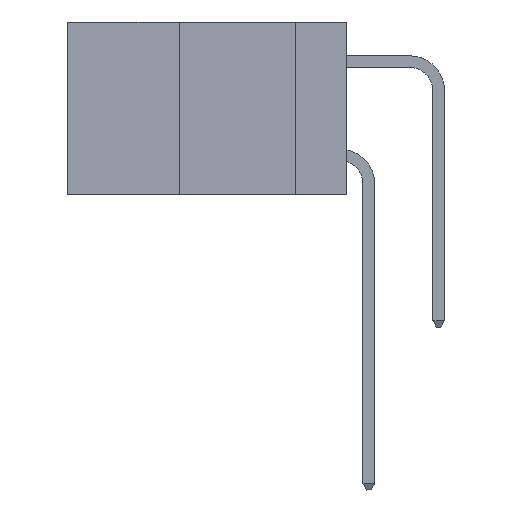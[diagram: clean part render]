
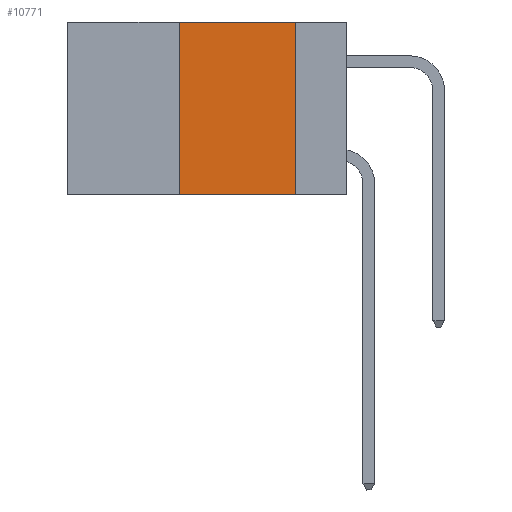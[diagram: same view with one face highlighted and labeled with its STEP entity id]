
A CAD part, left-side view. The second image highlights one B-rep face of the part: STEP entity #10771.
In plain terms, the highlighted planar face has unit normal (-1, 0, 0).
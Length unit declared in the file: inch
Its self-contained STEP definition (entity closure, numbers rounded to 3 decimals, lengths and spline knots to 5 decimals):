
#454 = VERTEX_POINT ( 'NONE', #17388 ) ;
#482 = PLANE ( 'NONE',  #4705 ) ;
#627 = EDGE_CURVE ( 'NONE', #16099, #19347, #20207, .T. ) ;
#819 = CARTESIAN_POINT ( 'NONE',  ( 0., 0.11, 0. ) ) ;
#1602 = CARTESIAN_POINT ( 'NONE',  ( 0., 0.11, -0.37 ) ) ;
#1875 = DIRECTION ( 'NONE',  ( 0., -1., 0. ) ) ;
#2126 = VECTOR ( 'NONE', #21507, 39.37008 ) ;
#2266 = DIRECTION ( 'NONE',  ( 1., 0., 0. ) ) ;
#2943 = EDGE_CURVE ( 'NONE', #454, #19347, #16893, .T. ) ;
#3566 = CARTESIAN_POINT ( 'NONE',  ( 0., 0.11, 0. ) ) ;
#4705 = AXIS2_PLACEMENT_3D ( 'NONE', #15575, #2266, #18907 ) ;
#5566 = ORIENTED_EDGE ( 'NONE', *, *, #17173, .F. ) ;
#5903 = ORIENTED_EDGE ( 'NONE', *, *, #627, .F. ) ;
#6256 = CARTESIAN_POINT ( 'NONE',  ( 0., 0.6, -0.37 ) ) ;
#6692 = LINE ( 'NONE', #11404, #2126 ) ;
#7516 = VECTOR ( 'NONE', #7964, 39.37008 ) ;
#7964 = DIRECTION ( 'NONE',  ( 0., -1., 0. ) ) ;
#8406 = FACE_OUTER_BOUND ( 'NONE', #18577, .T. ) ;
#9780 = ORIENTED_EDGE ( 'NONE', *, *, #2943, .T. ) ;
#10770 = VECTOR ( 'NONE', #16052, 39.37008 ) ;
#10771 = ADVANCED_FACE ( 'NONE', ( #8406 ), #482, .F. ) ;
#11404 = CARTESIAN_POINT ( 'NONE',  ( 0., 0.36, 0. ) ) ;
#13070 = LINE ( 'NONE', #13634, #14631 ) ;
#13322 = EDGE_CURVE ( 'NONE', #454, #16764, #6692, .T. ) ;
#13634 = CARTESIAN_POINT ( 'NONE',  ( 0., 0.6, 0. ) ) ;
#14631 = VECTOR ( 'NONE', #1875, 39.37008 ) ;
#15575 = CARTESIAN_POINT ( 'NONE',  ( 0., 0.6, 0. ) ) ;
#16052 = DIRECTION ( 'NONE',  ( 0., 0., -1. ) ) ;
#16099 = VERTEX_POINT ( 'NONE', #3566 ) ;
#16764 = VERTEX_POINT ( 'NONE', #20538 ) ;
#16893 = LINE ( 'NONE', #6256, #7516 ) ;
#17173 = EDGE_CURVE ( 'NONE', #16764, #16099, #13070, .T. ) ;
#17388 = CARTESIAN_POINT ( 'NONE',  ( 0., 0.36, -0.37 ) ) ;
#18476 = ORIENTED_EDGE ( 'NONE', *, *, #13322, .F. ) ;
#18577 = EDGE_LOOP ( 'NONE', ( #5903, #5566, #18476, #9780 ) ) ;
#18907 = DIRECTION ( 'NONE',  ( 0., 0., -1. ) ) ;
#19347 = VERTEX_POINT ( 'NONE', #1602 ) ;
#20207 = LINE ( 'NONE', #819, #10770 ) ;
#20538 = CARTESIAN_POINT ( 'NONE',  ( 0., 0.36, 0. ) ) ;
#21507 = DIRECTION ( 'NONE',  ( 0., 0., 1. ) ) ;
